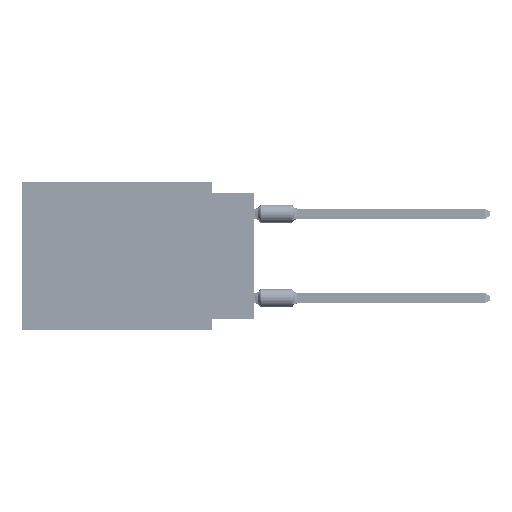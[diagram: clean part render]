
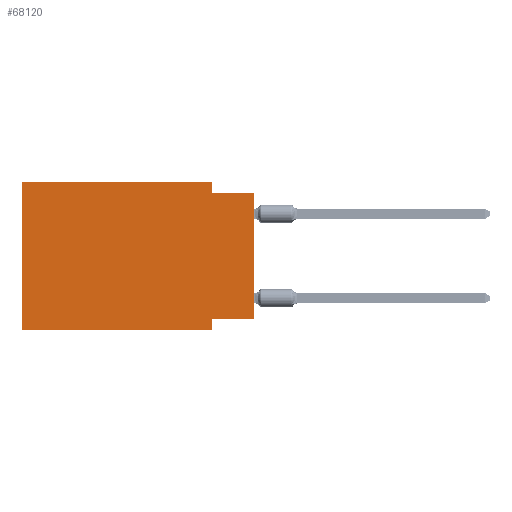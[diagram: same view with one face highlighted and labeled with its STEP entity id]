
A CAD part, left-side view. The second image highlights one B-rep face of the part: STEP entity #68120.
In plain terms, the highlighted planar face has unit normal (-1, 0, 0).
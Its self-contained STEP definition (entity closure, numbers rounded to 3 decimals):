
#5727 = VERTEX_POINT ( 'NONE', #35242 ) ;
#6683 = ORIENTED_EDGE ( 'NONE', *, *, #54969, .F. ) ;
#7575 = VECTOR ( 'NONE', #71054, 1000. ) ;
#7693 = EDGE_CURVE ( 'NONE', #27074, #21620, #53560, .T. ) ;
#9918 = VERTEX_POINT ( 'NONE', #54122 ) ;
#10347 = VERTEX_POINT ( 'NONE', #75679 ) ;
#12416 = VECTOR ( 'NONE', #64485, 1000. ) ;
#13331 = VERTEX_POINT ( 'NONE', #72663 ) ;
#15034 = DIRECTION ( 'NONE',  ( 0., -1., 0. ) ) ;
#15632 = VECTOR ( 'NONE', #51307, 1000. ) ;
#16600 = LINE ( 'NONE', #30550, #15632 ) ;
#18390 = DIRECTION ( 'NONE',  ( 0., 0., 1. ) ) ;
#20326 = EDGE_CURVE ( 'NONE', #13331, #9918, #21442, .T. ) ;
#21442 = LINE ( 'NONE', #48949, #7575 ) ;
#21620 = VERTEX_POINT ( 'NONE', #85503 ) ;
#22799 = VECTOR ( 'NONE', #18390, 1000. ) ;
#24752 = EDGE_CURVE ( 'NONE', #21620, #28289, #30775, .T. ) ;
#25933 = EDGE_CURVE ( 'NONE', #80428, #10347, #16600, .T. ) ;
#27074 = VERTEX_POINT ( 'NONE', #53098 ) ;
#27678 = LINE ( 'NONE', #67425, #68371 ) ;
#28097 = ORIENTED_EDGE ( 'NONE', *, *, #24752, .F. ) ;
#28289 = VERTEX_POINT ( 'NONE', #76619 ) ;
#30550 = CARTESIAN_POINT ( 'NONE',  ( 0., 0., 0. ) ) ;
#30775 = LINE ( 'NONE', #77740, #70251 ) ;
#31063 = CARTESIAN_POINT ( 'NONE',  ( 0., 0., -0.635 ) ) ;
#35242 = CARTESIAN_POINT ( 'NONE',  ( 0., 2.54, -0.635 ) ) ;
#35416 = VECTOR ( 'NONE', #65439, 1000. ) ;
#37888 = LINE ( 'NONE', #65879, #35416 ) ;
#38242 = DIRECTION ( 'NONE',  ( 0., 0., -1. ) ) ;
#41494 = EDGE_CURVE ( 'NONE', #80428, #13331, #73743, .T. ) ;
#44448 = DIRECTION ( 'NONE',  ( 0., 1., 0. ) ) ;
#45005 = CARTESIAN_POINT ( 'NONE',  ( 0., 13.97, 0. ) ) ;
#48949 = CARTESIAN_POINT ( 'NONE',  ( 0., 2.54, -8.89 ) ) ;
#51307 = DIRECTION ( 'NONE',  ( 0., 0., 1. ) ) ;
#52222 = PLANE ( 'NONE',  #64588 ) ;
#53098 = CARTESIAN_POINT ( 'NONE',  ( 0., 13.97, -8.89 ) ) ;
#53380 = EDGE_CURVE ( 'NONE', #27074, #9918, #27678, .T. ) ;
#53560 = LINE ( 'NONE', #81553, #22799 ) ;
#54122 = CARTESIAN_POINT ( 'NONE',  ( 0., 2.54, -8.89 ) ) ;
#54278 = ORIENTED_EDGE ( 'NONE', *, *, #7693, .F. ) ;
#54767 = DIRECTION ( 'NONE',  ( 0., -1., 0. ) ) ;
#54969 = EDGE_CURVE ( 'NONE', #28289, #5727, #37888, .T. ) ;
#56470 = ORIENTED_EDGE ( 'NONE', *, *, #65976, .F. ) ;
#60966 = ORIENTED_EDGE ( 'NONE', *, *, #53380, .T. ) ;
#64044 = LINE ( 'NONE', #31063, #12416 ) ;
#64485 = DIRECTION ( 'NONE',  ( 0., -1., 0. ) ) ;
#64588 = AXIS2_PLACEMENT_3D ( 'NONE', #45005, #72988, #38242 ) ;
#65234 = ORIENTED_EDGE ( 'NONE', *, *, #25933, .T. ) ;
#65439 = DIRECTION ( 'NONE',  ( 0., 0., -1. ) ) ;
#65879 = CARTESIAN_POINT ( 'NONE',  ( 0., 2.54, 0. ) ) ;
#65976 = EDGE_CURVE ( 'NONE', #5727, #10347, #64044, .T. ) ;
#67425 = CARTESIAN_POINT ( 'NONE',  ( 0., 13.97, -8.89 ) ) ;
#68120 = ADVANCED_FACE ( 'NONE', ( #79312 ), #52222, .F. ) ;
#68371 = VECTOR ( 'NONE', #54767, 1000. ) ;
#69715 = CARTESIAN_POINT ( 'NONE',  ( 0., 0., -8.255 ) ) ;
#70199 = VECTOR ( 'NONE', #44448, 1000. ) ;
#70251 = VECTOR ( 'NONE', #15034, 1000. ) ;
#71054 = DIRECTION ( 'NONE',  ( 0., 0., -1. ) ) ;
#71979 = CARTESIAN_POINT ( 'NONE',  ( 0., 0., -8.255 ) ) ;
#72663 = CARTESIAN_POINT ( 'NONE',  ( 0., 2.54, -8.255 ) ) ;
#72988 = DIRECTION ( 'NONE',  ( 1., 0., 0. ) ) ;
#73743 = LINE ( 'NONE', #71979, #70199 ) ;
#75679 = CARTESIAN_POINT ( 'NONE',  ( 0., 0., -0.635 ) ) ;
#76619 = CARTESIAN_POINT ( 'NONE',  ( 0., 2.54, 0. ) ) ;
#77740 = CARTESIAN_POINT ( 'NONE',  ( 0., 13.97, 0. ) ) ;
#78059 = ORIENTED_EDGE ( 'NONE', *, *, #41494, .F. ) ;
#79312 = FACE_OUTER_BOUND ( 'NONE', #86651, .T. ) ;
#80428 = VERTEX_POINT ( 'NONE', #69715 ) ;
#81553 = CARTESIAN_POINT ( 'NONE',  ( 0., 13.97, 0. ) ) ;
#85503 = CARTESIAN_POINT ( 'NONE',  ( 0., 13.97, 0. ) ) ;
#85617 = ORIENTED_EDGE ( 'NONE', *, *, #20326, .F. ) ;
#86651 = EDGE_LOOP ( 'NONE', ( #65234, #56470, #6683, #28097, #54278, #60966, #85617, #78059 ) ) ;
